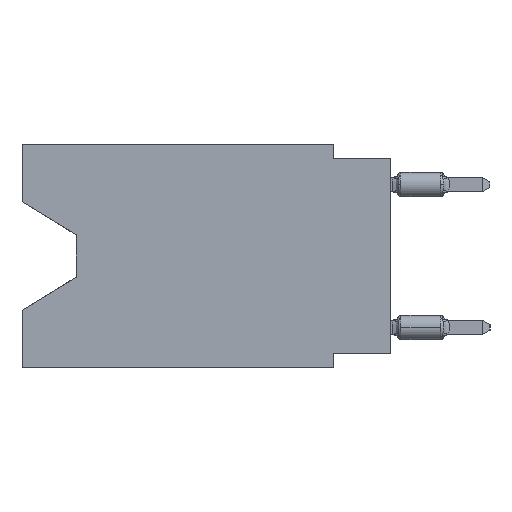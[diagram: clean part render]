
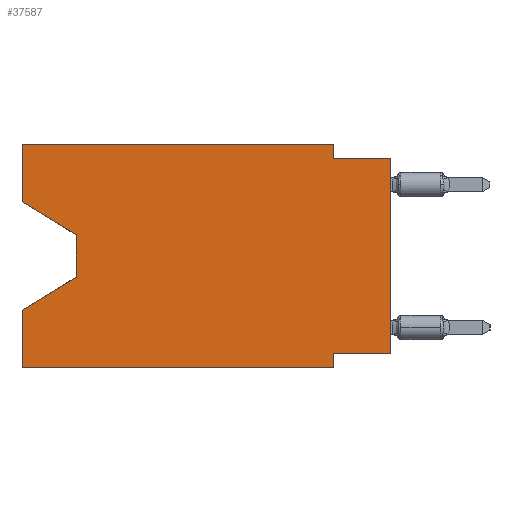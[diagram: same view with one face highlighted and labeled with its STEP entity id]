
A CAD part, left-side view. The second image highlights one B-rep face of the part: STEP entity #37587.
In plain terms, the highlighted planar face has unit normal (-1, 0, 0).
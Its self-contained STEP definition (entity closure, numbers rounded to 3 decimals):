
#1112 = LINE ( 'NONE', #28128, #5287 ) ;
#1158 = EDGE_CURVE ( 'NONE', #11620, #13135, #2465, .T. ) ;
#1234 = CARTESIAN_POINT ( 'NONE',  ( 0., 2.54, 0. ) ) ;
#1610 = FACE_OUTER_BOUND ( 'NONE', #26190, .T. ) ;
#2252 = LINE ( 'NONE', #12116, #6821 ) ;
#2465 = LINE ( 'NONE', #41955, #33884 ) ;
#3162 = VECTOR ( 'NONE', #16509, 1000. ) ;
#3172 = VECTOR ( 'NONE', #35133, 1000. ) ;
#3685 = DIRECTION ( 'NONE',  ( 0., 0., 1. ) ) ;
#5080 = CARTESIAN_POINT ( 'NONE',  ( 0., 2.54, -9.271 ) ) ;
#5269 = CARTESIAN_POINT ( 'NONE',  ( 0., 16.383, 0. ) ) ;
#5287 = VECTOR ( 'NONE', #34359, 1000. ) ;
#5456 = ORIENTED_EDGE ( 'NONE', *, *, #11275, .F. ) ;
#5876 = DIRECTION ( 'NONE',  ( 0., 0., -1. ) ) ;
#6378 = CARTESIAN_POINT ( 'NONE',  ( 0., 16.383, -9.906 ) ) ;
#6684 = CARTESIAN_POINT ( 'NONE',  ( 0., 16.383, 0. ) ) ;
#6821 = VECTOR ( 'NONE', #5876, 1000. ) ;
#7497 = VECTOR ( 'NONE', #3685, 1000. ) ;
#7818 = PLANE ( 'NONE',  #19209 ) ;
#8093 = VECTOR ( 'NONE', #37692, 1000. ) ;
#8541 = EDGE_CURVE ( 'NONE', #38816, #23970, #36090, .T. ) ;
#9077 = EDGE_CURVE ( 'NONE', #27282, #14112, #2252, .T. ) ;
#9316 = CARTESIAN_POINT ( 'NONE',  ( 0., 13.97, -5.893 ) ) ;
#9320 = DIRECTION ( 'NONE',  ( 0., 0., 1. ) ) ;
#9546 = ORIENTED_EDGE ( 'NONE', *, *, #8541, .F. ) ;
#11275 = EDGE_CURVE ( 'NONE', #36776, #40634, #38636, .T. ) ;
#11620 = VERTEX_POINT ( 'NONE', #6378 ) ;
#12116 = CARTESIAN_POINT ( 'NONE',  ( 0., 2.54, -9.906 ) ) ;
#12377 = CARTESIAN_POINT ( 'NONE',  ( 0., 0., 0. ) ) ;
#13135 = VERTEX_POINT ( 'NONE', #31873 ) ;
#13416 = ORIENTED_EDGE ( 'NONE', *, *, #41966, .F. ) ;
#14112 = VERTEX_POINT ( 'NONE', #16887 ) ;
#14617 = VERTEX_POINT ( 'NONE', #27348 ) ;
#15315 = ORIENTED_EDGE ( 'NONE', *, *, #33766, .T. ) ;
#16100 = VERTEX_POINT ( 'NONE', #36297 ) ;
#16171 = ORIENTED_EDGE ( 'NONE', *, *, #30745, .F. ) ;
#16509 = DIRECTION ( 'NONE',  ( 0., -0.855, -0.519 ) ) ;
#16518 = DIRECTION ( 'NONE',  ( 0., -1., 0. ) ) ;
#16887 = CARTESIAN_POINT ( 'NONE',  ( 0., 2.54, -9.906 ) ) ;
#17579 = ORIENTED_EDGE ( 'NONE', *, *, #1158, .F. ) ;
#18352 = VECTOR ( 'NONE', #30409, 1000. ) ;
#18976 = LINE ( 'NONE', #9316, #26621 ) ;
#19209 = AXIS2_PLACEMENT_3D ( 'NONE', #20711, #24146, #33813 ) ;
#19428 = EDGE_CURVE ( 'NONE', #11620, #14112, #36847, .T. ) ;
#19491 = EDGE_CURVE ( 'NONE', #23970, #24733, #34262, .T. ) ;
#19624 = DIRECTION ( 'NONE',  ( 0., 0.855, -0.519 ) ) ;
#20528 = CARTESIAN_POINT ( 'NONE',  ( 0., 13.97, -4.013 ) ) ;
#20530 = DIRECTION ( 'NONE',  ( 0., -1., 0. ) ) ;
#20711 = CARTESIAN_POINT ( 'NONE',  ( 0., 16.383, 0. ) ) ;
#20733 = CARTESIAN_POINT ( 'NONE',  ( 0., 16.383, -9.906 ) ) ;
#21124 = VECTOR ( 'NONE', #20530, 1000. ) ;
#21895 = LINE ( 'NONE', #34988, #3162 ) ;
#22748 = CARTESIAN_POINT ( 'NONE',  ( 0., 0., -0.635 ) ) ;
#22790 = LINE ( 'NONE', #26226, #36519 ) ;
#23040 = ORIENTED_EDGE ( 'NONE', *, *, #24144, .T. ) ;
#23970 = VERTEX_POINT ( 'NONE', #25736 ) ;
#24144 = EDGE_CURVE ( 'NONE', #38816, #14617, #21895, .T. ) ;
#24146 = DIRECTION ( 'NONE',  ( 1., 0., 0. ) ) ;
#24408 = CARTESIAN_POINT ( 'NONE',  ( 0., 16.383, -2.546 ) ) ;
#24733 = VERTEX_POINT ( 'NONE', #1234 ) ;
#25183 = VERTEX_POINT ( 'NONE', #28143 ) ;
#25736 = CARTESIAN_POINT ( 'NONE',  ( 0., 16.383, 0. ) ) ;
#26190 = EDGE_LOOP ( 'NONE', ( #23040, #27673, #15315, #17579, #35531, #35321, #13416, #36184, #5456, #16171, #40909, #9546 ) ) ;
#26226 = CARTESIAN_POINT ( 'NONE',  ( 0., 0., -9.271 ) ) ;
#26621 = VECTOR ( 'NONE', #19624, 1000. ) ;
#26805 = CARTESIAN_POINT ( 'NONE',  ( 0., 0., -0.635 ) ) ;
#27282 = VERTEX_POINT ( 'NONE', #5080 ) ;
#27348 = CARTESIAN_POINT ( 'NONE',  ( 0., 13.97, -4.013 ) ) ;
#27673 = ORIENTED_EDGE ( 'NONE', *, *, #33512, .T. ) ;
#28128 = CARTESIAN_POINT ( 'NONE',  ( 0., 2.54, 0. ) ) ;
#28143 = CARTESIAN_POINT ( 'NONE',  ( 0., 13.97, -5.893 ) ) ;
#30409 = DIRECTION ( 'NONE',  ( 0., 0., -1. ) ) ;
#30745 = EDGE_CURVE ( 'NONE', #24733, #36776, #1112, .T. ) ;
#31289 = EDGE_CURVE ( 'NONE', #16100, #40634, #35565, .T. ) ;
#31873 = CARTESIAN_POINT ( 'NONE',  ( 0., 16.383, -7.36 ) ) ;
#33512 = EDGE_CURVE ( 'NONE', #14617, #25183, #33836, .T. ) ;
#33766 = EDGE_CURVE ( 'NONE', #25183, #13135, #18976, .T. ) ;
#33813 = DIRECTION ( 'NONE',  ( 0., 0., -1. ) ) ;
#33836 = LINE ( 'NONE', #20528, #18352 ) ;
#33884 = VECTOR ( 'NONE', #9320, 1000. ) ;
#34262 = LINE ( 'NONE', #5269, #8093 ) ;
#34359 = DIRECTION ( 'NONE',  ( 0., 0., -1. ) ) ;
#34988 = CARTESIAN_POINT ( 'NONE',  ( 0., 16.383, -2.546 ) ) ;
#35133 = DIRECTION ( 'NONE',  ( 0., 0., 1. ) ) ;
#35211 = CARTESIAN_POINT ( 'NONE',  ( 0., 2.54, -0.635 ) ) ;
#35321 = ORIENTED_EDGE ( 'NONE', *, *, #9077, .F. ) ;
#35531 = ORIENTED_EDGE ( 'NONE', *, *, #19428, .T. ) ;
#35565 = LINE ( 'NONE', #12377, #3172 ) ;
#36090 = LINE ( 'NONE', #6684, #7497 ) ;
#36184 = ORIENTED_EDGE ( 'NONE', *, *, #31289, .T. ) ;
#36297 = CARTESIAN_POINT ( 'NONE',  ( 0., 0., -9.271 ) ) ;
#36519 = VECTOR ( 'NONE', #39330, 1000. ) ;
#36776 = VERTEX_POINT ( 'NONE', #35211 ) ;
#36847 = LINE ( 'NONE', #20733, #21124 ) ;
#37587 = ADVANCED_FACE ( 'NONE', ( #1610 ), #7818, .F. ) ;
#37692 = DIRECTION ( 'NONE',  ( 0., -1., 0. ) ) ;
#38636 = LINE ( 'NONE', #22748, #40591 ) ;
#38816 = VERTEX_POINT ( 'NONE', #24408 ) ;
#39330 = DIRECTION ( 'NONE',  ( 0., 1., 0. ) ) ;
#40591 = VECTOR ( 'NONE', #16518, 1000. ) ;
#40634 = VERTEX_POINT ( 'NONE', #26805 ) ;
#40909 = ORIENTED_EDGE ( 'NONE', *, *, #19491, .F. ) ;
#41955 = CARTESIAN_POINT ( 'NONE',  ( 0., 16.383, 0. ) ) ;
#41966 = EDGE_CURVE ( 'NONE', #16100, #27282, #22790, .T. ) ;
